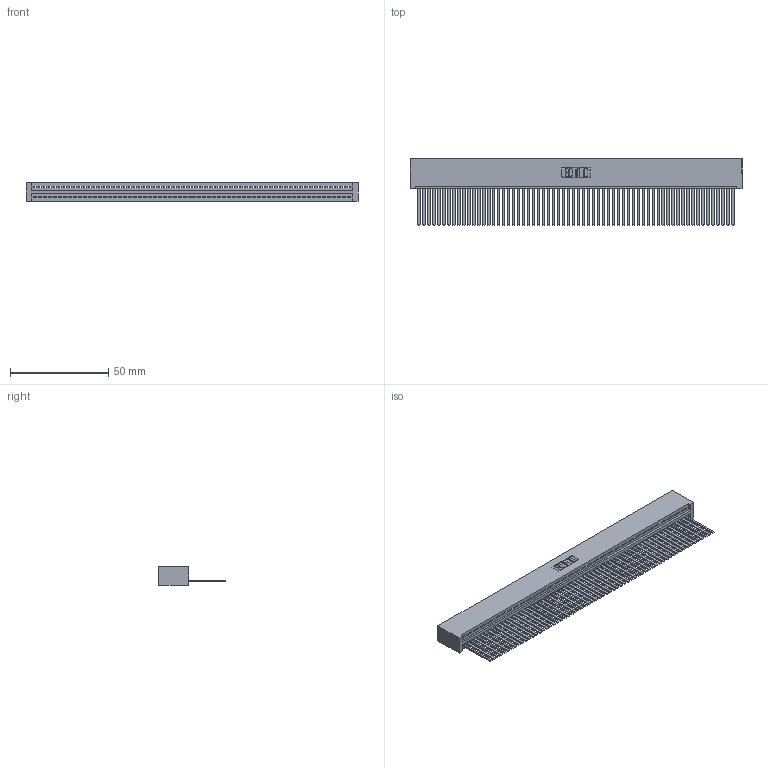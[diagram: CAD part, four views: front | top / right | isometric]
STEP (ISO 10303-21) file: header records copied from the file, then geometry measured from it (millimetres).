
FILE_DESCRIPTION (( 'STEP AP203' ), '1' );
FILE_NAME ('345-064-544-101.STEP', '2019-10-11T15:44:16', ( '' ), ( '' ), 'SwSTEP 2.0', 'SolidWorks 2016', '' );
FILE_SCHEMA (( 'CONFIG_CONTROL_DESIGN' ));
Length unit declared in the file: inch
Products named in the file (3): 345-064-544-101; 345-292-001_345-293-144; 345 Part_No Mounting Lugs
Assembly tree (65 placements, depth 2):
  345-064-544-101
    345 Part_No Mounting Lugs
    345-292-001_345-293-144  x64
Bounding box: 169.16 x 33.96 x 9.4 mm (x, y, z)
Volume: 17573.1 mm3; surface area: 26067.4 mm2
Topology: 65 solids, 65 shells, 3446 faces, 10429 edges, 6866 vertices
Faces by surface type: plane 2380, cylinder 1066
Entity records: 44745 total; most frequent: CARTESIAN_POINT 7756, ORIENTED_EDGE 7754, DIRECTION 6733, EDGE_CURVE 3877, LINE 3501, VECTOR 3501, VERTEX_POINT 2582, AXIS2_PLACEMENT_3D 1616
